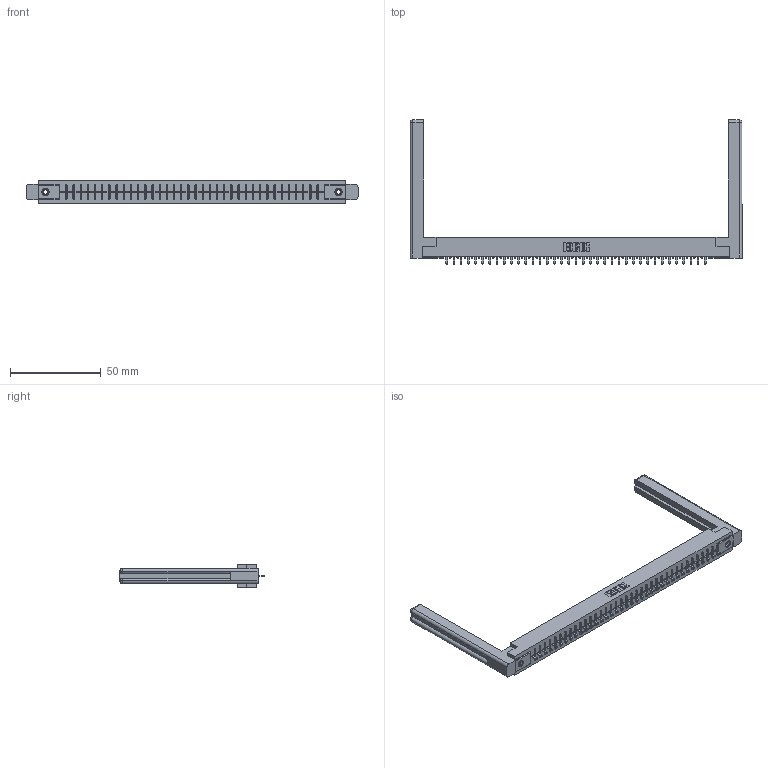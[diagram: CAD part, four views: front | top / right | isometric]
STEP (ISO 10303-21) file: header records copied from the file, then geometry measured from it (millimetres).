
FILE_DESCRIPTION (( 'STEP AP203' ), '1' );
FILE_NAME ('356-037-521-158.STEP', '2018-08-01T22:07:36', ( '' ), ( '' ), 'SwSTEP 2.0', 'SolidWorks 2016', '' );
FILE_SCHEMA (( 'CONFIG_CONTROL_DESIGN' ));
Length unit declared in the file: inch
Products named in the file (5): 306 Part_.156 Dia; 306-290-001_121; 345-250-001_345-250-001-102; 307-220-058; 356-037-521-158
Assembly tree (42 placements, depth 2):
  356-037-521-158
    306 Part_.156 Dia
    306-290-001_121  x37
    345-250-001_345-250-001-102  x2
    307-220-058  x2
Bounding box: 183.24 x 79.53 x 12.7 mm (x, y, z)
Volume: 27241.1 mm3; surface area: 25505.3 mm2
Topology: 42 solids, 42 shells, 2848 faces, 7959 edges, 5094 vertices
Faces by surface type: plane 1891, cylinder 785, sphere 148, cone 12, torus 12
Entity records: 37741 total; most frequent: CARTESIAN_POINT 6345, ORIENTED_EDGE 6232, DIRECTION 6212, EDGE_CURVE 3116, VECTOR 2430, LINE 2430, VERTEX_POINT 1970, AXIS2_PLACEMENT_3D 1891
